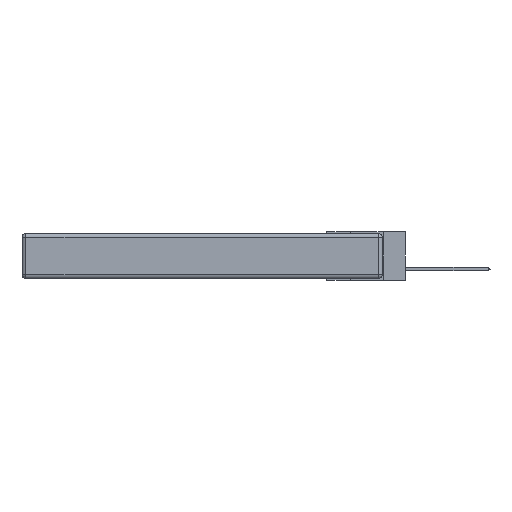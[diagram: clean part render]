
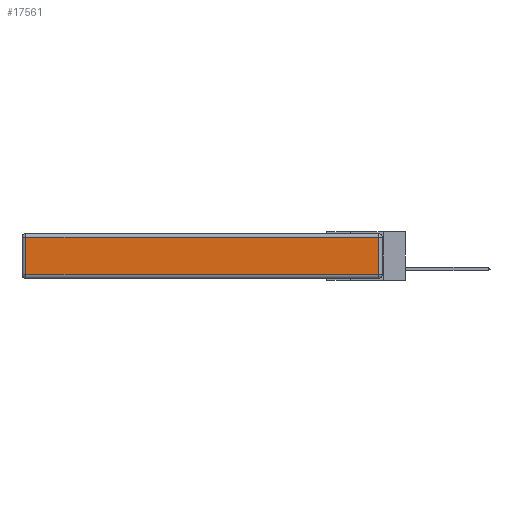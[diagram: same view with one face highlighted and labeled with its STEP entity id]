
A CAD part, left-side view. The second image highlights one B-rep face of the part: STEP entity #17561.
In plain terms, the highlighted planar face has unit normal (-1, 0, 0).
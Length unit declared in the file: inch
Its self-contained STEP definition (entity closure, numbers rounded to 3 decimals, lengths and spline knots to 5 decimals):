
#1003 = CARTESIAN_POINT ( 'NONE',  ( 0., 0.03, -0.343 ) ) ;
#1161 = EDGE_LOOP ( 'NONE', ( #19116, #11254, #12035, #10238 ) ) ;
#2013 = VECTOR ( 'NONE', #16407, 39.37008 ) ;
#2355 = CARTESIAN_POINT ( 'NONE',  ( 0., 2.72, -0.03 ) ) ;
#2577 = AXIS2_PLACEMENT_3D ( 'NONE', #14678, #12896, #3353 ) ;
#2781 = VERTEX_POINT ( 'NONE', #13268 ) ;
#3353 = DIRECTION ( 'NONE',  ( 0., 0., 1. ) ) ;
#3700 = EDGE_CURVE ( 'NONE', #6139, #2781, #7086, .T. ) ;
#4344 = DIRECTION ( 'NONE',  ( 0., 1., 0. ) ) ;
#5160 = LINE ( 'NONE', #8229, #13857 ) ;
#5664 = LINE ( 'NONE', #14129, #17403 ) ;
#5750 = EDGE_CURVE ( 'NONE', #22108, #17337, #5664, .T. ) ;
#6139 = VERTEX_POINT ( 'NONE', #24667 ) ;
#7086 = LINE ( 'NONE', #1003, #2013 ) ;
#8169 = EDGE_CURVE ( 'NONE', #17337, #6139, #17289, .T. ) ;
#8229 = CARTESIAN_POINT ( 'NONE',  ( 0., 2.75, -0.03 ) ) ;
#10238 = ORIENTED_EDGE ( 'NONE', *, *, #5750, .T. ) ;
#11254 = ORIENTED_EDGE ( 'NONE', *, *, #3700, .T. ) ;
#12035 = ORIENTED_EDGE ( 'NONE', *, *, #15930, .T. ) ;
#12036 = DIRECTION ( 'NONE',  ( 0., 0., -1. ) ) ;
#12896 = DIRECTION ( 'NONE',  ( -1., 0., 0. ) ) ;
#13268 = CARTESIAN_POINT ( 'NONE',  ( 0., 0.03, -0.03 ) ) ;
#13857 = VECTOR ( 'NONE', #4344, 39.37008 ) ;
#14129 = CARTESIAN_POINT ( 'NONE',  ( 0., 2.72, -0.343 ) ) ;
#14678 = CARTESIAN_POINT ( 'NONE',  ( 0., 0., -0.343 ) ) ;
#14731 = CARTESIAN_POINT ( 'NONE',  ( 0., 0., -0.313 ) ) ;
#15178 = VECTOR ( 'NONE', #22297, 39.37008 ) ;
#15930 = EDGE_CURVE ( 'NONE', #2781, #22108, #5160, .T. ) ;
#16407 = DIRECTION ( 'NONE',  ( 0., 0., 1. ) ) ;
#16470 = PLANE ( 'NONE',  #2577 ) ;
#17289 = LINE ( 'NONE', #14731, #15178 ) ;
#17337 = VERTEX_POINT ( 'NONE', #21008 ) ;
#17403 = VECTOR ( 'NONE', #12036, 39.37008 ) ;
#17561 = ADVANCED_FACE ( 'NONE', ( #17789 ), #16470, .T. ) ;
#17789 = FACE_OUTER_BOUND ( 'NONE', #1161, .T. ) ;
#19116 = ORIENTED_EDGE ( 'NONE', *, *, #8169, .T. ) ;
#21008 = CARTESIAN_POINT ( 'NONE',  ( 0., 2.72, -0.313 ) ) ;
#22108 = VERTEX_POINT ( 'NONE', #2355 ) ;
#22297 = DIRECTION ( 'NONE',  ( 0., -1., 0. ) ) ;
#24667 = CARTESIAN_POINT ( 'NONE',  ( 0., 0.03, -0.313 ) ) ;
